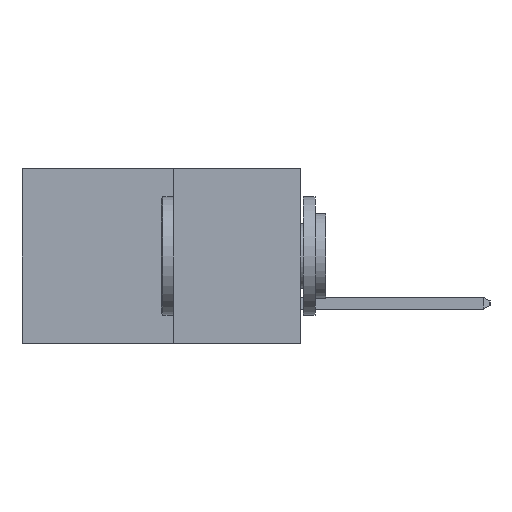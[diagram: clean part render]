
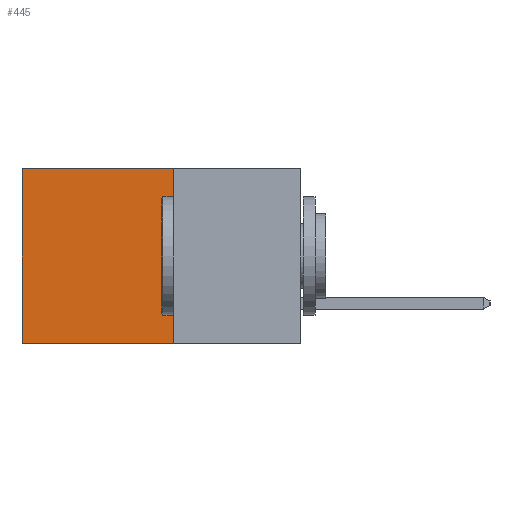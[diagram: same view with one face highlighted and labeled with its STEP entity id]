
A CAD part, left-side view. The second image highlights one B-rep face of the part: STEP entity #445.
In plain terms, the highlighted planar face has unit normal (-1, 0, 0).
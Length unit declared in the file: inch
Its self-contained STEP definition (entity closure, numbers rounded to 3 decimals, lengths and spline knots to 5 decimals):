
#77 = CARTESIAN_POINT ( 'NONE',  ( 0.277, 0.27, 0. ) ) ;
#225 = CARTESIAN_POINT ( 'NONE',  ( 0.277, 0.27, -0.37 ) ) ;
#445 = ADVANCED_FACE ( 'NONE', ( #16288 ), #4055, .F. ) ;
#754 = DIRECTION ( 'NONE',  ( 0., 0., -1. ) ) ;
#883 = DIRECTION ( 'NONE',  ( 1., 0., 0. ) ) ;
#3688 = CARTESIAN_POINT ( 'NONE',  ( 0.277, 0.59, 0. ) ) ;
#4055 = PLANE ( 'NONE',  #16273 ) ;
#4146 = VECTOR ( 'NONE', #11524, 39.37008 ) ;
#4376 = EDGE_CURVE ( 'NONE', #12892, #12884, #16258, .T. ) ;
#4419 = LINE ( 'NONE', #5826, #7864 ) ;
#4594 = ORIENTED_EDGE ( 'NONE', *, *, #14353, .T. ) ;
#4705 = DIRECTION ( 'NONE',  ( 0., 1., 0. ) ) ;
#4744 = CARTESIAN_POINT ( 'NONE',  ( 0.277, 0.27, -0.37 ) ) ;
#5545 = VECTOR ( 'NONE', #15427, 39.37008 ) ;
#5826 = CARTESIAN_POINT ( 'NONE',  ( 0.277, 0.59, -0.37 ) ) ;
#5830 = CARTESIAN_POINT ( 'NONE',  ( 0.277, 0.59, -0.37 ) ) ;
#5998 = EDGE_CURVE ( 'NONE', #10937, #10764, #7992, .T. ) ;
#7464 = ORIENTED_EDGE ( 'NONE', *, *, #7970, .F. ) ;
#7864 = VECTOR ( 'NONE', #14719, 39.37008 ) ;
#7970 = EDGE_CURVE ( 'NONE', #10937, #12892, #9403, .T. ) ;
#7992 = LINE ( 'NONE', #11585, #4146 ) ;
#9243 = ORIENTED_EDGE ( 'NONE', *, *, #5998, .T. ) ;
#9403 = LINE ( 'NONE', #10477, #5545 ) ;
#10477 = CARTESIAN_POINT ( 'NONE',  ( 0.277, 0.27, -0.37 ) ) ;
#10764 = VERTEX_POINT ( 'NONE', #3688 ) ;
#10937 = VERTEX_POINT ( 'NONE', #77 ) ;
#11018 = CARTESIAN_POINT ( 'NONE',  ( 0.277, 0.27, -0.37 ) ) ;
#11524 = DIRECTION ( 'NONE',  ( 0., 1., 0. ) ) ;
#11585 = CARTESIAN_POINT ( 'NONE',  ( 0.277, 0.27, 0. ) ) ;
#12359 = EDGE_LOOP ( 'NONE', ( #4594, #13256, #7464, #9243 ) ) ;
#12884 = VERTEX_POINT ( 'NONE', #5830 ) ;
#12892 = VERTEX_POINT ( 'NONE', #11018 ) ;
#13256 = ORIENTED_EDGE ( 'NONE', *, *, #4376, .F. ) ;
#14353 = EDGE_CURVE ( 'NONE', #10764, #12884, #4419, .T. ) ;
#14719 = DIRECTION ( 'NONE',  ( 0., 0., -1. ) ) ;
#15427 = DIRECTION ( 'NONE',  ( 0., 0., -1. ) ) ;
#15881 = VECTOR ( 'NONE', #4705, 39.37008 ) ;
#16258 = LINE ( 'NONE', #4744, #15881 ) ;
#16273 = AXIS2_PLACEMENT_3D ( 'NONE', #225, #883, #754 ) ;
#16288 = FACE_OUTER_BOUND ( 'NONE', #12359, .T. ) ;
